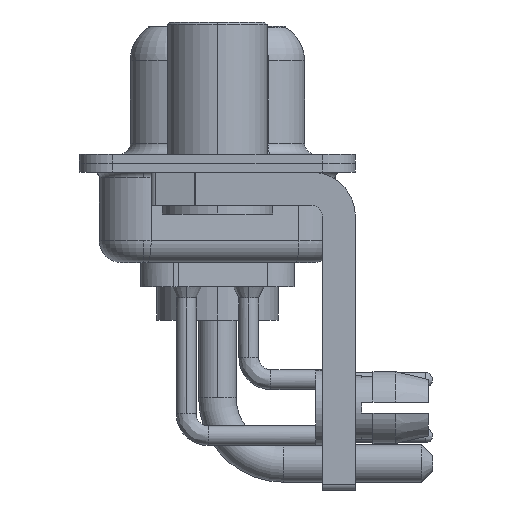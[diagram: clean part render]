
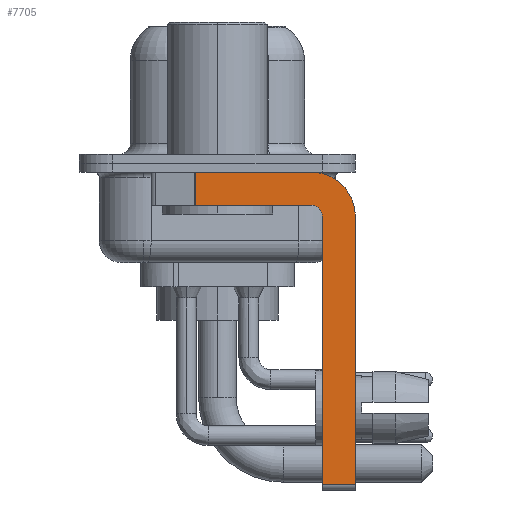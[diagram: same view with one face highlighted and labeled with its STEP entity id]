
A CAD part, left-side view. The second image highlights one B-rep face of the part: STEP entity #7705.
In plain terms, the highlighted planar face has unit normal (-1, 0, 0).
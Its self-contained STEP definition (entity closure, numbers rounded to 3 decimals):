
#837 = DIRECTION ( 'NONE',  ( 0., 0., 1. ) ) ;
#1218 = VECTOR ( 'NONE', #10519, 1000. ) ;
#1424 = DIRECTION ( 'NONE',  ( 0., -1., 0. ) ) ;
#1437 = CARTESIAN_POINT ( 'NONE',  ( -2.9, -4.25, -2.4 ) ) ;
#1458 = ORIENTED_EDGE ( 'NONE', *, *, #5311, .T. ) ;
#1557 = VECTOR ( 'NONE', #9857, 1000. ) ;
#2314 = VECTOR ( 'NONE', #8460, 1000. ) ;
#3496 = LINE ( 'NONE', #15506, #1218 ) ;
#3778 = CARTESIAN_POINT ( 'NONE',  ( -2.9, -4.75, -14.55 ) ) ;
#4064 = CIRCLE ( 'NONE', #17555, 0.5 ) ;
#4157 = EDGE_CURVE ( 'NONE', #9692, #15210, #12745, .T. ) ;
#4425 = CARTESIAN_POINT ( 'NONE',  ( -2.9, -6.25, -2.4 ) ) ;
#4611 = CIRCLE ( 'NONE', #12094, 2. ) ;
#4836 = CARTESIAN_POINT ( 'NONE',  ( -2.9, -6.25, -2.4 ) ) ;
#4899 = DIRECTION ( 'NONE',  ( 1., 0., 0. ) ) ;
#4974 = FACE_OUTER_BOUND ( 'NONE', #9334, .T. ) ;
#5311 = EDGE_CURVE ( 'NONE', #12231, #8626, #9805, .T. ) ;
#5696 = ORIENTED_EDGE ( 'NONE', *, *, #11422, .F. ) ;
#6641 = CARTESIAN_POINT ( 'NONE',  ( -2.9, -4.25, -2.4 ) ) ;
#6680 = CARTESIAN_POINT ( 'NONE',  ( -2.9, 0.978, -1.9 ) ) ;
#7212 = VERTEX_POINT ( 'NONE', #17939 ) ;
#7432 = ORIENTED_EDGE ( 'NONE', *, *, #8966, .F. ) ;
#7705 = ADVANCED_FACE ( 'NONE', ( #4974 ), #18540, .F. ) ;
#7724 = CARTESIAN_POINT ( 'NONE',  ( -2.9, -4.25, -0.4 ) ) ;
#7762 = CARTESIAN_POINT ( 'NONE',  ( -2.9, 0.978, -0.4 ) ) ;
#8058 = EDGE_CURVE ( 'NONE', #7212, #9692, #4064, .T. ) ;
#8460 = DIRECTION ( 'NONE',  ( 0., -1., 0. ) ) ;
#8507 = LINE ( 'NONE', #4836, #1557 ) ;
#8626 = VERTEX_POINT ( 'NONE', #8872 ) ;
#8872 = CARTESIAN_POINT ( 'NONE',  ( -2.9, -6.25, -14.55 ) ) ;
#8966 = EDGE_CURVE ( 'NONE', #12363, #17937, #15134, .T. ) ;
#9334 = EDGE_LOOP ( 'NONE', ( #7432, #12791, #14223, #11692, #5696, #1458, #19444, #10433 ) ) ;
#9659 = VECTOR ( 'NONE', #12314, 1000. ) ;
#9692 = VERTEX_POINT ( 'NONE', #15434 ) ;
#9794 = VECTOR ( 'NONE', #12125, 1000. ) ;
#9805 = LINE ( 'NONE', #19777, #16739 ) ;
#9857 = DIRECTION ( 'NONE',  ( 0., 0., -1. ) ) ;
#10433 = ORIENTED_EDGE ( 'NONE', *, *, #18539, .F. ) ;
#10519 = DIRECTION ( 'NONE',  ( 0., 0., 1. ) ) ;
#11198 = CARTESIAN_POINT ( 'NONE',  ( -2.9, -4.25, -2.4 ) ) ;
#11266 = EDGE_CURVE ( 'NONE', #12668, #8626, #8507, .T. ) ;
#11422 = EDGE_CURVE ( 'NONE', #12231, #7212, #3496, .T. ) ;
#11462 = CARTESIAN_POINT ( 'NONE',  ( -2.9, 3., -0.4 ) ) ;
#11552 = DIRECTION ( 'NONE',  ( 1., 0., 0. ) ) ;
#11692 = ORIENTED_EDGE ( 'NONE', *, *, #8058, .F. ) ;
#11923 = DIRECTION ( 'NONE',  ( 0., 0., -1. ) ) ;
#12094 = AXIS2_PLACEMENT_3D ( 'NONE', #1437, #4899, #11923 ) ;
#12125 = DIRECTION ( 'NONE',  ( 0., 0., -1. ) ) ;
#12231 = VERTEX_POINT ( 'NONE', #3778 ) ;
#12314 = DIRECTION ( 'NONE',  ( 0., 1., 0. ) ) ;
#12331 = EDGE_CURVE ( 'NONE', #12363, #15210, #20556, .T. ) ;
#12363 = VERTEX_POINT ( 'NONE', #7762 ) ;
#12668 = VERTEX_POINT ( 'NONE', #4425 ) ;
#12745 = LINE ( 'NONE', #17407, #9659 ) ;
#12791 = ORIENTED_EDGE ( 'NONE', *, *, #12331, .T. ) ;
#13441 = DIRECTION ( 'NONE',  ( 0., 0., -1. ) ) ;
#14223 = ORIENTED_EDGE ( 'NONE', *, *, #4157, .F. ) ;
#15134 = LINE ( 'NONE', #11462, #2314 ) ;
#15210 = VERTEX_POINT ( 'NONE', #6680 ) ;
#15397 = AXIS2_PLACEMENT_3D ( 'NONE', #6641, #11552, #13441 ) ;
#15434 = CARTESIAN_POINT ( 'NONE',  ( -2.9, -4.25, -1.9 ) ) ;
#15506 = CARTESIAN_POINT ( 'NONE',  ( -2.9, -4.75, -14.8 ) ) ;
#16739 = VECTOR ( 'NONE', #1424, 1000. ) ;
#17407 = CARTESIAN_POINT ( 'NONE',  ( -2.9, -4.25, -1.9 ) ) ;
#17555 = AXIS2_PLACEMENT_3D ( 'NONE', #11198, #18071, #837 ) ;
#17937 = VERTEX_POINT ( 'NONE', #7724 ) ;
#17939 = CARTESIAN_POINT ( 'NONE',  ( -2.9, -4.75, -2.4 ) ) ;
#18071 = DIRECTION ( 'NONE',  ( -1., 0., 0. ) ) ;
#18539 = EDGE_CURVE ( 'NONE', #17937, #12668, #4611, .T. ) ;
#18540 = PLANE ( 'NONE',  #15397 ) ;
#19444 = ORIENTED_EDGE ( 'NONE', *, *, #11266, .F. ) ;
#19777 = CARTESIAN_POINT ( 'NONE',  ( -2.9, -4.25, -14.55 ) ) ;
#20556 = LINE ( 'NONE', #21978, #9794 ) ;
#21978 = CARTESIAN_POINT ( 'NONE',  ( -2.9, 0.978, -1.9 ) ) ;
